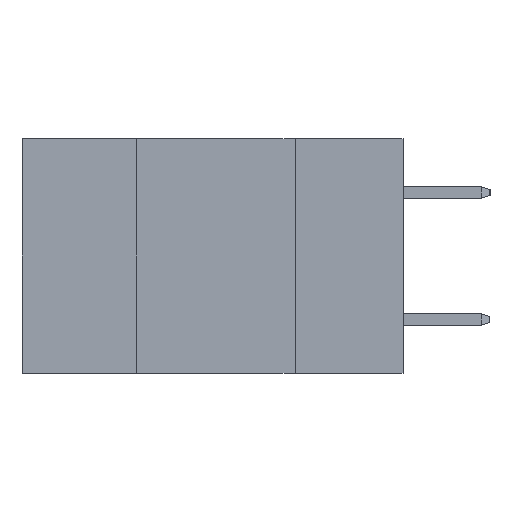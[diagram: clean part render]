
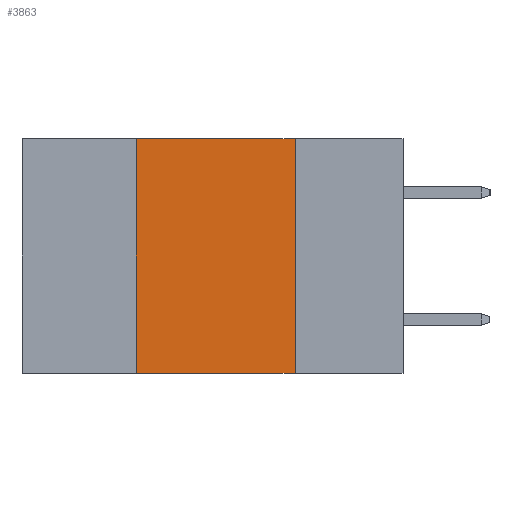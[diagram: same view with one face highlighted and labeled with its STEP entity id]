
A CAD part, left-side view. The second image highlights one B-rep face of the part: STEP entity #3863.
In plain terms, the highlighted planar face has unit normal (-1, 0, 0).
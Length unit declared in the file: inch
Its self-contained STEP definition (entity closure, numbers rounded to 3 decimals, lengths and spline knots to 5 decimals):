
#35 = DIRECTION ( 'NONE',  ( 0., 0., -1. ) ) ;
#99 = LINE ( 'NONE', #607, #9676 ) ;
#144 = ORIENTED_EDGE ( 'NONE', *, *, #10803, .F. ) ;
#234 = ORIENTED_EDGE ( 'NONE', *, *, #3355, .F. ) ;
#278 = DIRECTION ( 'NONE',  ( 0., 0., 1. ) ) ;
#607 = CARTESIAN_POINT ( 'NONE',  ( 0., 0.6, -0.37 ) ) ;
#1455 = EDGE_CURVE ( 'NONE', #4669, #5748, #11211, .T. ) ;
#1640 = DIRECTION ( 'NONE',  ( 0., -1., 0. ) ) ;
#1887 = PLANE ( 'NONE',  #10901 ) ;
#2764 = DIRECTION ( 'NONE',  ( 0., 0., -1. ) ) ;
#2981 = LINE ( 'NONE', #6615, #6433 ) ;
#3355 = EDGE_CURVE ( 'NONE', #5748, #3864, #2981, .T. ) ;
#3863 = ADVANCED_FACE ( 'NONE', ( #5324 ), #1887, .F. ) ;
#3864 = VERTEX_POINT ( 'NONE', #7160 ) ;
#4626 = DIRECTION ( 'NONE',  ( 0., -1., 0. ) ) ;
#4669 = VERTEX_POINT ( 'NONE', #4875 ) ;
#4875 = CARTESIAN_POINT ( 'NONE',  ( 0., 0.42, -0.37 ) ) ;
#5005 = CARTESIAN_POINT ( 'NONE',  ( 0., 0.42, 0. ) ) ;
#5324 = FACE_OUTER_BOUND ( 'NONE', #10189, .T. ) ;
#5423 = CARTESIAN_POINT ( 'NONE',  ( 0., 0.17, 0. ) ) ;
#5748 = VERTEX_POINT ( 'NONE', #7059 ) ;
#6391 = LINE ( 'NONE', #5423, #7959 ) ;
#6433 = VECTOR ( 'NONE', #1640, 39.37008 ) ;
#6615 = CARTESIAN_POINT ( 'NONE',  ( 0., 0.6, 0. ) ) ;
#6740 = EDGE_CURVE ( 'NONE', #4669, #8734, #99, .T. ) ;
#7059 = CARTESIAN_POINT ( 'NONE',  ( 0., 0.42, 0. ) ) ;
#7160 = CARTESIAN_POINT ( 'NONE',  ( 0., 0.17, 0. ) ) ;
#7341 = DIRECTION ( 'NONE',  ( 1., 0., 0. ) ) ;
#7959 = VECTOR ( 'NONE', #2764, 39.37008 ) ;
#8219 = ORIENTED_EDGE ( 'NONE', *, *, #6740, .T. ) ;
#8451 = VECTOR ( 'NONE', #278, 39.37008 ) ;
#8734 = VERTEX_POINT ( 'NONE', #9637 ) ;
#8850 = ORIENTED_EDGE ( 'NONE', *, *, #1455, .F. ) ;
#8924 = CARTESIAN_POINT ( 'NONE',  ( 0., 0.6, 0. ) ) ;
#9637 = CARTESIAN_POINT ( 'NONE',  ( 0., 0.17, -0.37 ) ) ;
#9676 = VECTOR ( 'NONE', #4626, 39.37008 ) ;
#10189 = EDGE_LOOP ( 'NONE', ( #144, #234, #8850, #8219 ) ) ;
#10803 = EDGE_CURVE ( 'NONE', #3864, #8734, #6391, .T. ) ;
#10901 = AXIS2_PLACEMENT_3D ( 'NONE', #8924, #7341, #35 ) ;
#11211 = LINE ( 'NONE', #5005, #8451 ) ;
